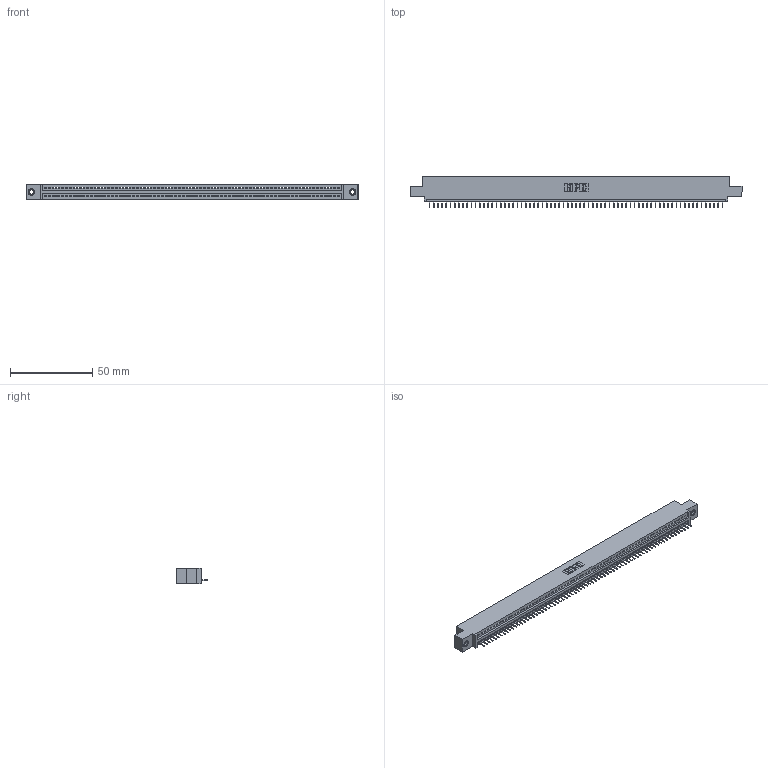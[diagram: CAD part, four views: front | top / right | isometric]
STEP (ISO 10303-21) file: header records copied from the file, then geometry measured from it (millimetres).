
FILE_DESCRIPTION (( 'STEP AP203' ), '1' );
FILE_NAME ('345-071-524-407.STEP', '2018-10-01T14:06:54', ( '' ), ( '' ), 'SwSTEP 2.0', 'SolidWorks 2016', '' );
FILE_SCHEMA (( 'CONFIG_CONTROL_DESIGN' ));
Length unit declared in the file: inch
Products named in the file (4): 345-292-001_345-293-124; 345-250-001_345-250-005-103; 345 Part_0.110 Offset - 0.156 Dia-TI; 345-071-524-407
Assembly tree (74 placements, depth 2):
  345-071-524-407
    345 Part_0.110 Offset - 0.156 Dia-TI
    345-292-001_345-293-124  x71
    345-250-001_345-250-005-103  x2
Bounding box: 201.55 x 19.35 x 9.4 mm (x, y, z)
Volume: 19013.5 mm3; surface area: 24879.1 mm2
Topology: 74 solids, 74 shells, 4592 faces, 13269 edges, 8554 vertices
Faces by surface type: plane 3382, cylinder 1194, cone 12, torus 4
Entity records: 50924 total; most frequent: CARTESIAN_POINT 8800, ORIENTED_EDGE 8798, DIRECTION 7671, EDGE_CURVE 4399, LINE 3967, VECTOR 3967, VERTEX_POINT 2924, AXIS2_PLACEMENT_3D 1852
